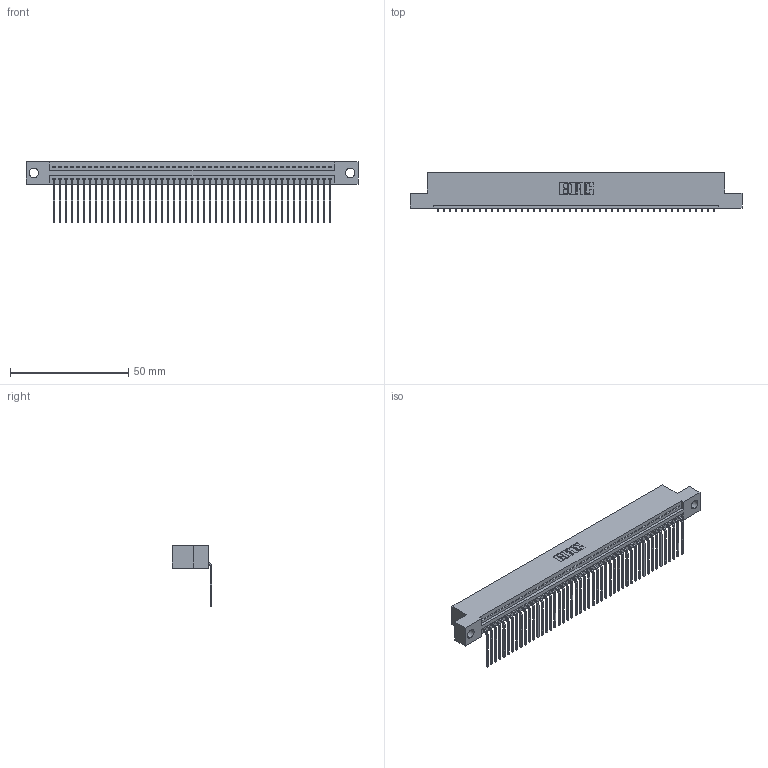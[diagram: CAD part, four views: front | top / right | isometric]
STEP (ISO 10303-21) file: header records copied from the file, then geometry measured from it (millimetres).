
FILE_DESCRIPTION (( 'STEP AP203' ), '1' );
FILE_NAME ('395-047-559-104.STEP', '2019-10-23T00:25:56', ( '' ), ( '' ), 'SwSTEP 2.0', 'SolidWorks 2016', '' );
FILE_SCHEMA (( 'CONFIG_CONTROL_DESIGN' ));
Length unit declared in the file: inch
Products named in the file (3): 345-292-001_558 559 Tail - 1; 395-047-559-104; 345 Part_Flush Mounting Lugs - 0.156 Dia-TH
Assembly tree (48 placements, depth 2):
  395-047-559-104
    345 Part_Flush Mounting Lugs - 0.156 Dia-TH
    345-292-001_558 559 Tail - 1  x47
Bounding box: 140.59 x 16.75 x 25.53 mm (x, y, z)
Volume: 13463 mm3; surface area: 18688 mm2
Topology: 48 solids, 48 shells, 2946 faces, 8895 edges, 5866 vertices
Faces by surface type: plane 2054, cylinder 892
Entity records: 34787 total; most frequent: CARTESIAN_POINT 6033, ORIENTED_EDGE 6014, DIRECTION 5261, EDGE_CURVE 3007, VECTOR 2687, LINE 2687, VERTEX_POINT 2002, AXIS2_PLACEMENT_3D 1287
